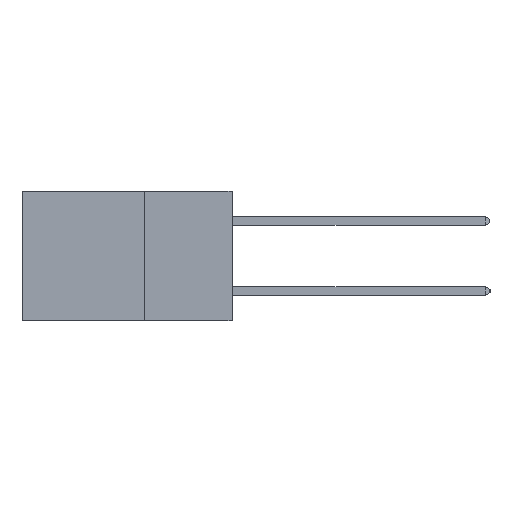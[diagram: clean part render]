
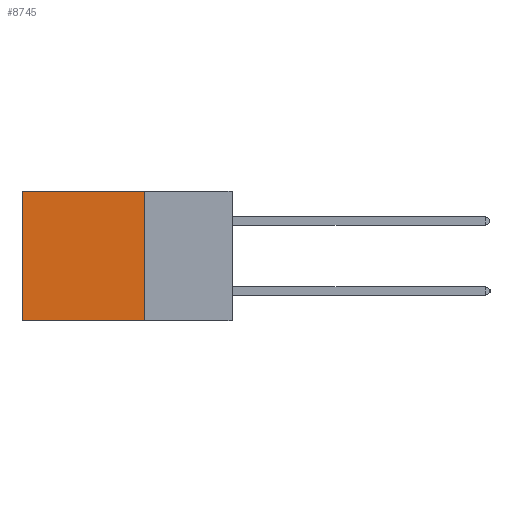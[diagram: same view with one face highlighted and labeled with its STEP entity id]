
A CAD part, left-side view. The second image highlights one B-rep face of the part: STEP entity #8745.
In plain terms, the highlighted planar face has unit normal (-1, 0, 0).
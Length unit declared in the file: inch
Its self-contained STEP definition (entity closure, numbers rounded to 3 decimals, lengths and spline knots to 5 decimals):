
#199 = FACE_OUTER_BOUND ( 'NONE', #3461, .T. ) ;
#1853 = EDGE_CURVE ( 'NONE', #16150, #12222, #19088, .T. ) ;
#3070 = LINE ( 'NONE', #8121, #20685 ) ;
#3094 = LINE ( 'NONE', #13788, #12299 ) ;
#3461 = EDGE_LOOP ( 'NONE', ( #8573, #6289, #5148, #13426 ) ) ;
#5148 = ORIENTED_EDGE ( 'NONE', *, *, #13994, .F. ) ;
#5763 = VERTEX_POINT ( 'NONE', #15140 ) ;
#6289 = ORIENTED_EDGE ( 'NONE', *, *, #14762, .F. ) ;
#6625 = DIRECTION ( 'NONE',  ( 0., 0., -1. ) ) ;
#7861 = CARTESIAN_POINT ( 'NONE',  ( 0.2875, 0.25, 0. ) ) ;
#8121 = CARTESIAN_POINT ( 'NONE',  ( 0.2875, 0.25, 0. ) ) ;
#8226 = EDGE_CURVE ( 'NONE', #5763, #16150, #3070, .T. ) ;
#8280 = CARTESIAN_POINT ( 'NONE',  ( 0.2875, 0.25, 0. ) ) ;
#8573 = ORIENTED_EDGE ( 'NONE', *, *, #1853, .T. ) ;
#8611 = DIRECTION ( 'NONE',  ( 0., 1., 0. ) ) ;
#8745 = ADVANCED_FACE ( 'NONE', ( #199 ), #18073, .F. ) ;
#9586 = DIRECTION ( 'NONE',  ( 0., 0., -1. ) ) ;
#12222 = VERTEX_POINT ( 'NONE', #14922 ) ;
#12299 = VECTOR ( 'NONE', #8611, 39.37008 ) ;
#12767 = CARTESIAN_POINT ( 'NONE',  ( 0.2875, 0.25, -0.37 ) ) ;
#12794 = DIRECTION ( 'NONE',  ( 0., 0., -1. ) ) ;
#13323 = DIRECTION ( 'NONE',  ( 0., 1., 0. ) ) ;
#13426 = ORIENTED_EDGE ( 'NONE', *, *, #8226, .T. ) ;
#13788 = CARTESIAN_POINT ( 'NONE',  ( 0.2875, 0.25, -0.37 ) ) ;
#13994 = EDGE_CURVE ( 'NONE', #5763, #15001, #21503, .T. ) ;
#14600 = AXIS2_PLACEMENT_3D ( 'NONE', #7861, #19769, #9586 ) ;
#14631 = VECTOR ( 'NONE', #12794, 39.37008 ) ;
#14762 = EDGE_CURVE ( 'NONE', #15001, #12222, #3094, .T. ) ;
#14922 = CARTESIAN_POINT ( 'NONE',  ( 0.2875, 0.6, -0.37 ) ) ;
#15001 = VERTEX_POINT ( 'NONE', #12767 ) ;
#15140 = CARTESIAN_POINT ( 'NONE',  ( 0.2875, 0.25, 0. ) ) ;
#15861 = CARTESIAN_POINT ( 'NONE',  ( 0.2875, 0.6, 0. ) ) ;
#16150 = VERTEX_POINT ( 'NONE', #15861 ) ;
#18073 = PLANE ( 'NONE',  #14600 ) ;
#18834 = CARTESIAN_POINT ( 'NONE',  ( 0.2875, 0.6, 0. ) ) ;
#19088 = LINE ( 'NONE', #18834, #14631 ) ;
#19769 = DIRECTION ( 'NONE',  ( 1., 0., 0. ) ) ;
#20685 = VECTOR ( 'NONE', #13323, 39.37008 ) ;
#20963 = VECTOR ( 'NONE', #6625, 39.37008 ) ;
#21503 = LINE ( 'NONE', #8280, #20963 ) ;
